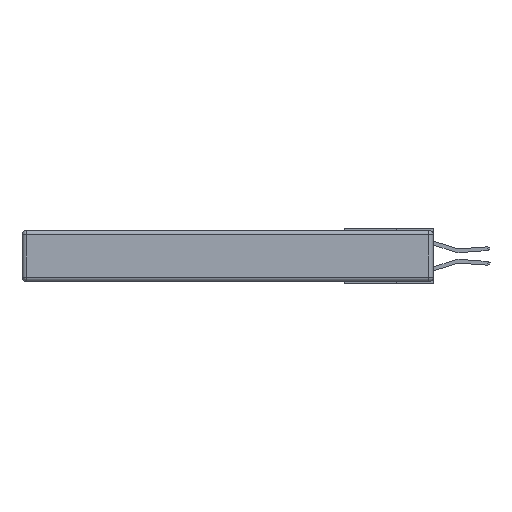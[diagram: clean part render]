
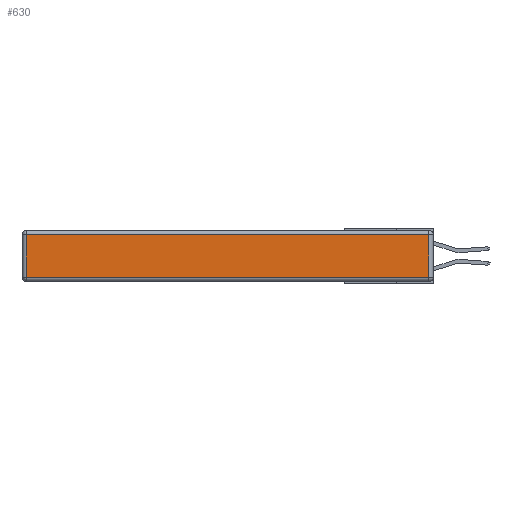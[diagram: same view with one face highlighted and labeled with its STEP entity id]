
A CAD part, left-side view. The second image highlights one B-rep face of the part: STEP entity #630.
In plain terms, the highlighted planar face has unit normal (-1, 0, 0).
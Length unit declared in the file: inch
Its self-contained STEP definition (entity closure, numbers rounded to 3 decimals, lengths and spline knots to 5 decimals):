
#260 = DIRECTION ( 'NONE',  ( 0., 0., -1. ) ) ;
#630 = ADVANCED_FACE ( 'NONE', ( #1496 ), #13928, .T. ) ;
#882 = CARTESIAN_POINT ( 'NONE',  ( 0., 0., -0.343 ) ) ;
#1172 = ORIENTED_EDGE ( 'NONE', *, *, #8413, .T. ) ;
#1459 = LINE ( 'NONE', #13222, #14082 ) ;
#1496 = FACE_OUTER_BOUND ( 'NONE', #5102, .T. ) ;
#1594 = CARTESIAN_POINT ( 'NONE',  ( 0., 0., -0.313 ) ) ;
#1605 = VECTOR ( 'NONE', #2883, 39.37008 ) ;
#1709 = VERTEX_POINT ( 'NONE', #6571 ) ;
#2668 = LINE ( 'NONE', #1594, #13902 ) ;
#2718 = CARTESIAN_POINT ( 'NONE',  ( 0., 0.03, -0.343 ) ) ;
#2883 = DIRECTION ( 'NONE',  ( 0., 0., 1. ) ) ;
#4165 = DIRECTION ( 'NONE',  ( 0., 1., 0. ) ) ;
#4352 = CARTESIAN_POINT ( 'NONE',  ( 0., 2.75, -0.03 ) ) ;
#4432 = VERTEX_POINT ( 'NONE', #4687 ) ;
#4687 = CARTESIAN_POINT ( 'NONE',  ( 0., 2.72, -0.03 ) ) ;
#4718 = CARTESIAN_POINT ( 'NONE',  ( 0., 2.72, -0.313 ) ) ;
#5102 = EDGE_LOOP ( 'NONE', ( #8963, #1172, #10221, #7314 ) ) ;
#5875 = DIRECTION ( 'NONE',  ( 0., -1., 0. ) ) ;
#6571 = CARTESIAN_POINT ( 'NONE',  ( 0., 0.03, -0.03 ) ) ;
#7094 = AXIS2_PLACEMENT_3D ( 'NONE', #882, #12839, #12796 ) ;
#7268 = VECTOR ( 'NONE', #4165, 39.37008 ) ;
#7314 = ORIENTED_EDGE ( 'NONE', *, *, #10590, .T. ) ;
#8327 = EDGE_CURVE ( 'NONE', #1709, #4432, #12528, .T. ) ;
#8413 = EDGE_CURVE ( 'NONE', #11622, #1709, #10292, .T. ) ;
#8963 = ORIENTED_EDGE ( 'NONE', *, *, #10788, .T. ) ;
#10221 = ORIENTED_EDGE ( 'NONE', *, *, #8327, .T. ) ;
#10292 = LINE ( 'NONE', #2718, #1605 ) ;
#10590 = EDGE_CURVE ( 'NONE', #4432, #12371, #1459, .T. ) ;
#10788 = EDGE_CURVE ( 'NONE', #12371, #11622, #2668, .T. ) ;
#11622 = VERTEX_POINT ( 'NONE', #13155 ) ;
#12371 = VERTEX_POINT ( 'NONE', #4718 ) ;
#12528 = LINE ( 'NONE', #4352, #7268 ) ;
#12796 = DIRECTION ( 'NONE',  ( 0., 0., 1. ) ) ;
#12839 = DIRECTION ( 'NONE',  ( -1., 0., 0. ) ) ;
#13155 = CARTESIAN_POINT ( 'NONE',  ( 0., 0.03, -0.313 ) ) ;
#13222 = CARTESIAN_POINT ( 'NONE',  ( 0., 2.72, -0.343 ) ) ;
#13902 = VECTOR ( 'NONE', #5875, 39.37008 ) ;
#13928 = PLANE ( 'NONE',  #7094 ) ;
#14082 = VECTOR ( 'NONE', #260, 39.37008 ) ;
